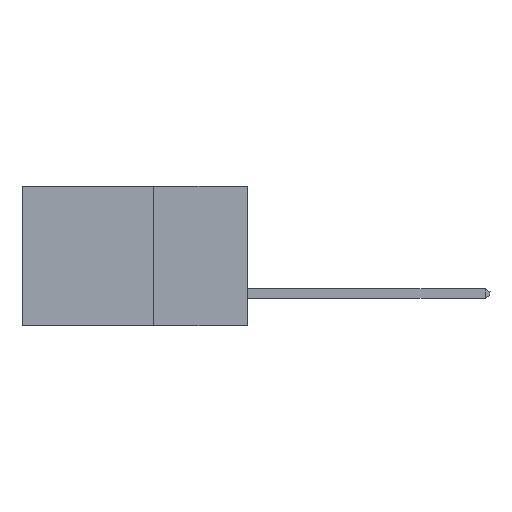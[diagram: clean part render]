
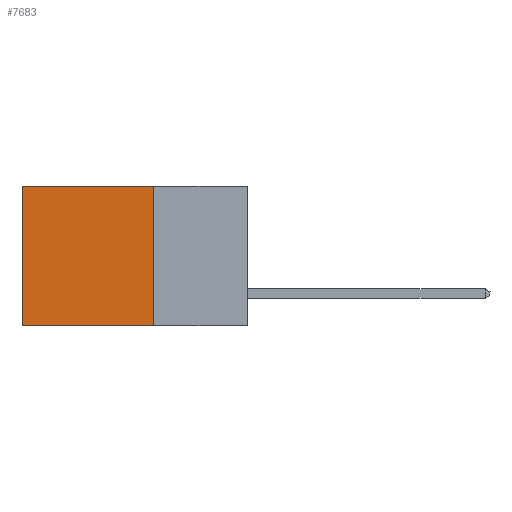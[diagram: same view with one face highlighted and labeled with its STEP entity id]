
A CAD part, left-side view. The second image highlights one B-rep face of the part: STEP entity #7683.
In plain terms, the highlighted planar face has unit normal (-1, 0, 0).
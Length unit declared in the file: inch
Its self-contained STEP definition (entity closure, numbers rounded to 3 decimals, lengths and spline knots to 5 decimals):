
#664 = CARTESIAN_POINT ( 'NONE',  ( 0.2615, 0.25, -0.37 ) ) ;
#798 = ORIENTED_EDGE ( 'NONE', *, *, #2618, .T. ) ;
#1414 = DIRECTION ( 'NONE',  ( 0., 1., 0. ) ) ;
#1622 = CARTESIAN_POINT ( 'NONE',  ( 0.2615, 0.6, 0. ) ) ;
#1976 = AXIS2_PLACEMENT_3D ( 'NONE', #10319, #2870, #6057 ) ;
#2126 = FACE_OUTER_BOUND ( 'NONE', #3233, .T. ) ;
#2138 = LINE ( 'NONE', #6116, #4452 ) ;
#2474 = VERTEX_POINT ( 'NONE', #4455 ) ;
#2618 = EDGE_CURVE ( 'NONE', #8414, #10183, #10415, .T. ) ;
#2870 = DIRECTION ( 'NONE',  ( 1., 0., 0. ) ) ;
#2912 = EDGE_CURVE ( 'NONE', #2474, #8414, #5278, .T. ) ;
#3120 = DIRECTION ( 'NONE',  ( 0., 0., -1. ) ) ;
#3233 = EDGE_LOOP ( 'NONE', ( #798, #7630, #6482, #8288 ) ) ;
#3604 = VECTOR ( 'NONE', #7090, 39.37008 ) ;
#3776 = DIRECTION ( 'NONE',  ( 0., 0., -1. ) ) ;
#4213 = CARTESIAN_POINT ( 'NONE',  ( 0.2615, 0.25, -0.37 ) ) ;
#4452 = VECTOR ( 'NONE', #3776, 39.37008 ) ;
#4455 = CARTESIAN_POINT ( 'NONE',  ( 0.2615, 0.25, 0. ) ) ;
#4547 = VERTEX_POINT ( 'NONE', #4213 ) ;
#4664 = EDGE_CURVE ( 'NONE', #2474, #4547, #2138, .T. ) ;
#4854 = CARTESIAN_POINT ( 'NONE',  ( 0.2615, 0.6, -0.37 ) ) ;
#5278 = LINE ( 'NONE', #5331, #6529 ) ;
#5331 = CARTESIAN_POINT ( 'NONE',  ( 0.2615, 0.25, 0. ) ) ;
#5481 = EDGE_CURVE ( 'NONE', #4547, #10183, #8667, .T. ) ;
#6057 = DIRECTION ( 'NONE',  ( 0., 0., -1. ) ) ;
#6116 = CARTESIAN_POINT ( 'NONE',  ( 0.2615, 0.25, -0.37 ) ) ;
#6482 = ORIENTED_EDGE ( 'NONE', *, *, #4664, .F. ) ;
#6529 = VECTOR ( 'NONE', #1414, 39.37008 ) ;
#7090 = DIRECTION ( 'NONE',  ( 0., 1., 0. ) ) ;
#7630 = ORIENTED_EDGE ( 'NONE', *, *, #5481, .F. ) ;
#7683 = ADVANCED_FACE ( 'NONE', ( #2126 ), #10154, .F. ) ;
#8161 = CARTESIAN_POINT ( 'NONE',  ( 0.2615, 0.6, -0.37 ) ) ;
#8288 = ORIENTED_EDGE ( 'NONE', *, *, #2912, .T. ) ;
#8407 = VECTOR ( 'NONE', #3120, 39.37008 ) ;
#8414 = VERTEX_POINT ( 'NONE', #1622 ) ;
#8667 = LINE ( 'NONE', #664, #3604 ) ;
#10154 = PLANE ( 'NONE',  #1976 ) ;
#10183 = VERTEX_POINT ( 'NONE', #4854 ) ;
#10319 = CARTESIAN_POINT ( 'NONE',  ( 0.2615, 0.25, -0.37 ) ) ;
#10415 = LINE ( 'NONE', #8161, #8407 ) ;
